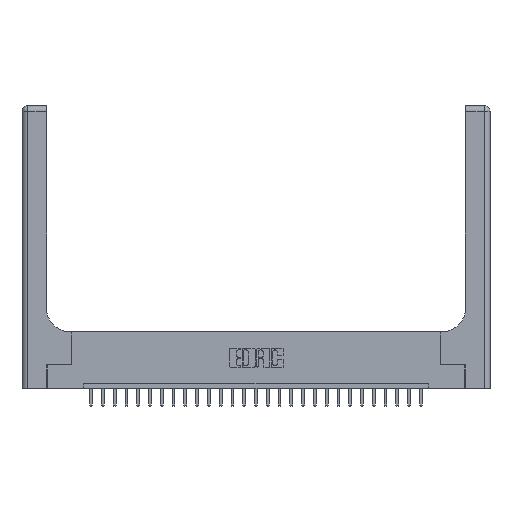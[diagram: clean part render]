
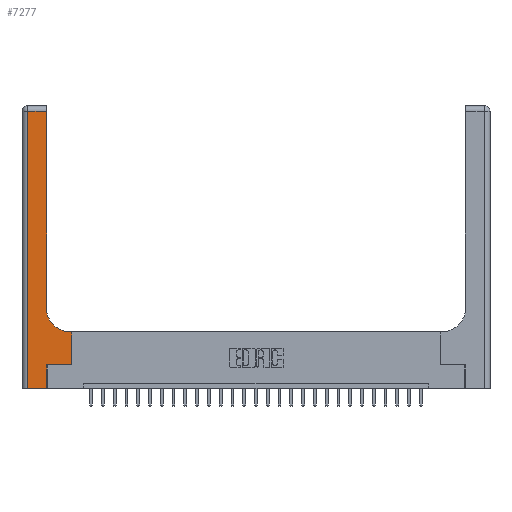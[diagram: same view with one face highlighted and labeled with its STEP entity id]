
A CAD part, top view. The second image highlights one B-rep face of the part: STEP entity #7277.
In plain terms, the highlighted planar face has unit normal (0, 0, 1).
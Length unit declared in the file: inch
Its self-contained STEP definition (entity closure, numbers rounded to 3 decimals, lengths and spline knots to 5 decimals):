
#17 = CARTESIAN_POINT ( 'NONE',  ( 0., 3., 0.37 ) ) ;
#47 = EDGE_CURVE ( 'NONE', #19213, #20209, #24707, .T. ) ;
#82 = VERTEX_POINT ( 'NONE', #18477 ) ;
#325 = CARTESIAN_POINT ( 'NONE',  ( 0.265, 0.25, 0.37 ) ) ;
#858 = EDGE_CURVE ( 'NONE', #5463, #10992, #20226, .T. ) ;
#1163 = CARTESIAN_POINT ( 'NONE',  ( 0.26, 0.6, 0.37 ) ) ;
#1221 = CARTESIAN_POINT ( 'NONE',  ( 0.265, 0.25, 0.37 ) ) ;
#1241 = DIRECTION ( 'NONE',  ( -1., 0., 0. ) ) ;
#1374 = CARTESIAN_POINT ( 'NONE',  ( 0.51, 0.85, 0.37 ) ) ;
#1658 = CARTESIAN_POINT ( 'NONE',  ( 0.26, 0.85, 0.37 ) ) ;
#1672 = CARTESIAN_POINT ( 'NONE',  ( 0.26, 2.94, 0.37 ) ) ;
#2002 = DIRECTION ( 'NONE',  ( 1., 0., 0. ) ) ;
#2106 = LINE ( 'NONE', #6120, #18492 ) ;
#2218 = CARTESIAN_POINT ( 'NONE',  ( 0., 0., 0.37 ) ) ;
#2716 = CARTESIAN_POINT ( 'NONE',  ( 0.265, 0., 0.37 ) ) ;
#3645 = CARTESIAN_POINT ( 'NONE',  ( 0.528, 0.25, 0.37 ) ) ;
#4438 = VECTOR ( 'NONE', #11230, 39.37008 ) ;
#4770 = AXIS2_PLACEMENT_3D ( 'NONE', #1374, #15025, #14943 ) ;
#5246 = VECTOR ( 'NONE', #2002, 39.37008 ) ;
#5463 = VERTEX_POINT ( 'NONE', #9332 ) ;
#6120 = CARTESIAN_POINT ( 'NONE',  ( 0., 2.94, 0.37 ) ) ;
#6365 = ORIENTED_EDGE ( 'NONE', *, *, #24145, .T. ) ;
#6369 = DIRECTION ( 'NONE',  ( 0., -1., 0. ) ) ;
#7205 = FACE_OUTER_BOUND ( 'NONE', #7253, .T. ) ;
#7253 = EDGE_LOOP ( 'NONE', ( #12228, #14611, #6365, #9143, #12317, #23251, #12176, #15738, #13123 ) ) ;
#7277 = ADVANCED_FACE ( 'NONE', ( #7205 ), #13688, .F. ) ;
#8417 = DIRECTION ( 'NONE',  ( 0., 1., 0. ) ) ;
#9143 = ORIENTED_EDGE ( 'NONE', *, *, #9737, .T. ) ;
#9313 = CIRCLE ( 'NONE', #4770, 0.25 ) ;
#9332 = CARTESIAN_POINT ( 'NONE',  ( 0.528, 0.6, 0.37 ) ) ;
#9737 = EDGE_CURVE ( 'NONE', #82, #11821, #18730, .T. ) ;
#10207 = VERTEX_POINT ( 'NONE', #16458 ) ;
#10234 = CARTESIAN_POINT ( 'NONE',  ( 0.265, 0., 0.37 ) ) ;
#10249 = VECTOR ( 'NONE', #11567, 39.37008 ) ;
#10431 = LINE ( 'NONE', #325, #5246 ) ;
#10450 = VERTEX_POINT ( 'NONE', #3645 ) ;
#10992 = VERTEX_POINT ( 'NONE', #19307 ) ;
#11230 = DIRECTION ( 'NONE',  ( 0., 1., 0. ) ) ;
#11567 = DIRECTION ( 'NONE',  ( 0., 1., 0. ) ) ;
#11666 = DIRECTION ( 'NONE',  ( 0., 0., -1. ) ) ;
#11821 = VERTEX_POINT ( 'NONE', #2716 ) ;
#12097 = CARTESIAN_POINT ( 'NONE',  ( 0.06, 3., 0.37 ) ) ;
#12176 = ORIENTED_EDGE ( 'NONE', *, *, #24495, .T. ) ;
#12228 = ORIENTED_EDGE ( 'NONE', *, *, #47, .T. ) ;
#12317 = ORIENTED_EDGE ( 'NONE', *, *, #19659, .T. ) ;
#12843 = CARTESIAN_POINT ( 'NONE',  ( 0.26, 3., 0.37 ) ) ;
#13123 = ORIENTED_EDGE ( 'NONE', *, *, #15479, .T. ) ;
#13619 = VECTOR ( 'NONE', #13709, 39.37008 ) ;
#13688 = PLANE ( 'NONE',  #23657 ) ;
#13709 = DIRECTION ( 'NONE',  ( 1., 0., 0. ) ) ;
#14611 = ORIENTED_EDGE ( 'NONE', *, *, #19361, .T. ) ;
#14943 = DIRECTION ( 'NONE',  ( 1., 0., 0. ) ) ;
#15025 = DIRECTION ( 'NONE',  ( 0., 0., -1. ) ) ;
#15378 = LINE ( 'NONE', #23281, #10249 ) ;
#15479 = EDGE_CURVE ( 'NONE', #10992, #19213, #9313, .T. ) ;
#15660 = VECTOR ( 'NONE', #6369, 39.37008 ) ;
#15738 = ORIENTED_EDGE ( 'NONE', *, *, #858, .T. ) ;
#16458 = CARTESIAN_POINT ( 'NONE',  ( 0.06, 2.94, 0.37 ) ) ;
#17730 = EDGE_CURVE ( 'NONE', #18511, #10450, #10431, .T. ) ;
#17888 = LINE ( 'NONE', #10234, #23606 ) ;
#18060 = VECTOR ( 'NONE', #1241, 39.37008 ) ;
#18477 = CARTESIAN_POINT ( 'NONE',  ( 0.06, 0., 0.37 ) ) ;
#18492 = VECTOR ( 'NONE', #23947, 39.37008 ) ;
#18511 = VERTEX_POINT ( 'NONE', #1221 ) ;
#18699 = LINE ( 'NONE', #12097, #15660 ) ;
#18730 = LINE ( 'NONE', #2218, #13619 ) ;
#19213 = VERTEX_POINT ( 'NONE', #1658 ) ;
#19307 = CARTESIAN_POINT ( 'NONE',  ( 0.51, 0.6, 0.37 ) ) ;
#19361 = EDGE_CURVE ( 'NONE', #20209, #10207, #2106, .T. ) ;
#19431 = DIRECTION ( 'NONE',  ( -1., 0., 0. ) ) ;
#19659 = EDGE_CURVE ( 'NONE', #11821, #18511, #17888, .T. ) ;
#20209 = VERTEX_POINT ( 'NONE', #1672 ) ;
#20226 = LINE ( 'NONE', #1163, #18060 ) ;
#23251 = ORIENTED_EDGE ( 'NONE', *, *, #17730, .T. ) ;
#23281 = CARTESIAN_POINT ( 'NONE',  ( 0.528, 0.25, 0.37 ) ) ;
#23606 = VECTOR ( 'NONE', #8417, 39.37008 ) ;
#23657 = AXIS2_PLACEMENT_3D ( 'NONE', #17, #11666, #19431 ) ;
#23947 = DIRECTION ( 'NONE',  ( -1., 0., 0. ) ) ;
#24145 = EDGE_CURVE ( 'NONE', #10207, #82, #18699, .T. ) ;
#24495 = EDGE_CURVE ( 'NONE', #10450, #5463, #15378, .T. ) ;
#24707 = LINE ( 'NONE', #12843, #4438 ) ;
